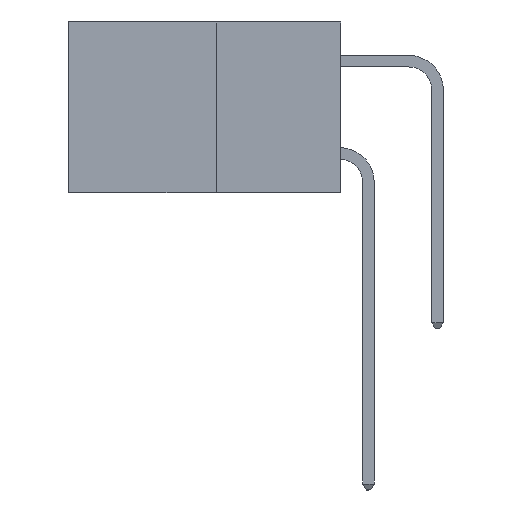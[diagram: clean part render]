
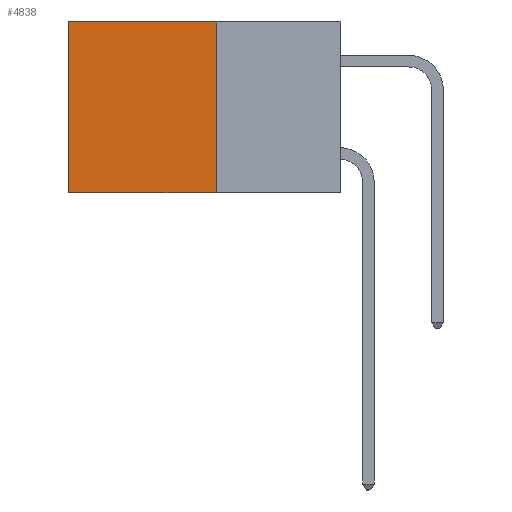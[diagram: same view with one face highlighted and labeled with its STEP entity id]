
A CAD part, left-side view. The second image highlights one B-rep face of the part: STEP entity #4838.
In plain terms, the highlighted planar face has unit normal (-1, 0, 0).
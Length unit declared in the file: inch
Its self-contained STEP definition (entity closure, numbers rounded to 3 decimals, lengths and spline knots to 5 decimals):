
#546 = LINE ( 'NONE', #11480, #7099 ) ;
#670 = VERTEX_POINT ( 'NONE', #8045 ) ;
#763 = DIRECTION ( 'NONE',  ( 1., 0., 0. ) ) ;
#803 = PLANE ( 'NONE',  #7372 ) ;
#873 = CARTESIAN_POINT ( 'NONE',  ( 0.277, 0.59, 0. ) ) ;
#1076 = VERTEX_POINT ( 'NONE', #9882 ) ;
#1126 = LINE ( 'NONE', #4024, #8218 ) ;
#1591 = ORIENTED_EDGE ( 'NONE', *, *, #9532, .F. ) ;
#1775 = VECTOR ( 'NONE', #6149, 39.37008 ) ;
#2463 = VECTOR ( 'NONE', #9102, 39.37008 ) ;
#3049 = ORIENTED_EDGE ( 'NONE', *, *, #11026, .T. ) ;
#3261 = ORIENTED_EDGE ( 'NONE', *, *, #7283, .F. ) ;
#3915 = ORIENTED_EDGE ( 'NONE', *, *, #7191, .T. ) ;
#4024 = CARTESIAN_POINT ( 'NONE',  ( 0.277, 0.59, -0.37 ) ) ;
#4838 = ADVANCED_FACE ( 'NONE', ( #10668 ), #803, .F. ) ;
#4959 = DIRECTION ( 'NONE',  ( 0., 0., -1. ) ) ;
#5288 = CARTESIAN_POINT ( 'NONE',  ( 0.277, 0.27, -0.37 ) ) ;
#5422 = CARTESIAN_POINT ( 'NONE',  ( 0.277, 0.27, -0.37 ) ) ;
#6149 = DIRECTION ( 'NONE',  ( 0., 1., 0. ) ) ;
#6882 = VERTEX_POINT ( 'NONE', #873 ) ;
#7099 = VECTOR ( 'NONE', #9685, 39.37008 ) ;
#7191 = EDGE_CURVE ( 'NONE', #6882, #670, #1126, .T. ) ;
#7283 = EDGE_CURVE ( 'NONE', #1076, #11557, #546, .T. ) ;
#7289 = DIRECTION ( 'NONE',  ( 0., 0., -1. ) ) ;
#7372 = AXIS2_PLACEMENT_3D ( 'NONE', #5422, #763, #7289 ) ;
#8045 = CARTESIAN_POINT ( 'NONE',  ( 0.277, 0.59, -0.37 ) ) ;
#8218 = VECTOR ( 'NONE', #4959, 39.37008 ) ;
#8864 = LINE ( 'NONE', #11590, #1775 ) ;
#9102 = DIRECTION ( 'NONE',  ( 0., 1., 0. ) ) ;
#9532 = EDGE_CURVE ( 'NONE', #11557, #670, #8864, .T. ) ;
#9685 = DIRECTION ( 'NONE',  ( 0., 0., -1. ) ) ;
#9882 = CARTESIAN_POINT ( 'NONE',  ( 0.277, 0.27, 0. ) ) ;
#10097 = LINE ( 'NONE', #10884, #2463 ) ;
#10668 = FACE_OUTER_BOUND ( 'NONE', #11781, .T. ) ;
#10884 = CARTESIAN_POINT ( 'NONE',  ( 0.277, 0.27, 0. ) ) ;
#11026 = EDGE_CURVE ( 'NONE', #1076, #6882, #10097, .T. ) ;
#11480 = CARTESIAN_POINT ( 'NONE',  ( 0.277, 0.27, -0.37 ) ) ;
#11557 = VERTEX_POINT ( 'NONE', #5288 ) ;
#11590 = CARTESIAN_POINT ( 'NONE',  ( 0.277, 0.27, -0.37 ) ) ;
#11781 = EDGE_LOOP ( 'NONE', ( #3915, #1591, #3261, #3049 ) ) ;
